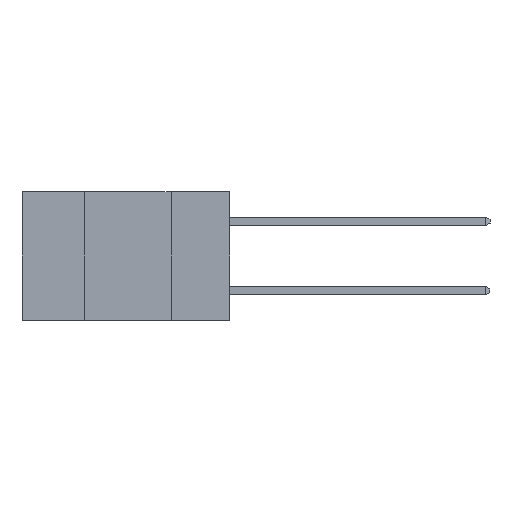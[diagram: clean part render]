
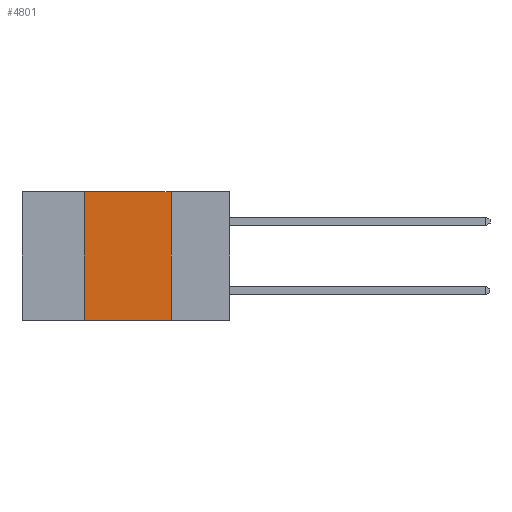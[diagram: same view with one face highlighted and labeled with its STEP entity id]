
A CAD part, left-side view. The second image highlights one B-rep face of the part: STEP entity #4801.
In plain terms, the highlighted planar face has unit normal (-1, 0, 0).
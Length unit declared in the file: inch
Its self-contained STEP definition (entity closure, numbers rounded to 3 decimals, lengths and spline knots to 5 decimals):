
#1340 = DIRECTION ( 'NONE',  ( 0., 0., -1. ) ) ;
#1509 = FACE_OUTER_BOUND ( 'NONE', #3841, .T. ) ;
#3841 = EDGE_LOOP ( 'NONE', ( #6502, #13847, #8459, #9207 ) ) ;
#3978 = VECTOR ( 'NONE', #1340, 39.37008 ) ;
#4552 = LINE ( 'NONE', #22559, #3978 ) ;
#4801 = ADVANCED_FACE ( 'NONE', ( #1509 ), #14738, .F. ) ;
#5911 = DIRECTION ( 'NONE',  ( 0., 0., 1. ) ) ;
#6206 = VERTEX_POINT ( 'NONE', #13933 ) ;
#6502 = ORIENTED_EDGE ( 'NONE', *, *, #14186, .F. ) ;
#7762 = CARTESIAN_POINT ( 'NONE',  ( 0., 0.42, -0.37 ) ) ;
#8459 = ORIENTED_EDGE ( 'NONE', *, *, #12145, .F. ) ;
#8888 = AXIS2_PLACEMENT_3D ( 'NONE', #14660, #15686, #22134 ) ;
#8908 = LINE ( 'NONE', #13937, #13091 ) ;
#9137 = CARTESIAN_POINT ( 'NONE',  ( 0., 0.17, 0. ) ) ;
#9207 = ORIENTED_EDGE ( 'NONE', *, *, #18111, .T. ) ;
#10358 = CARTESIAN_POINT ( 'NONE',  ( 0., 0.42, 0. ) ) ;
#10503 = VERTEX_POINT ( 'NONE', #10358 ) ;
#10595 = EDGE_CURVE ( 'NONE', #10503, #22707, #19248, .T. ) ;
#12145 = EDGE_CURVE ( 'NONE', #13924, #10503, #13664, .T. ) ;
#12261 = DIRECTION ( 'NONE',  ( 0., -1., 0. ) ) ;
#13091 = VECTOR ( 'NONE', #12261, 39.37008 ) ;
#13664 = LINE ( 'NONE', #20096, #17794 ) ;
#13847 = ORIENTED_EDGE ( 'NONE', *, *, #10595, .F. ) ;
#13924 = VERTEX_POINT ( 'NONE', #7762 ) ;
#13933 = CARTESIAN_POINT ( 'NONE',  ( 0., 0.17, -0.37 ) ) ;
#13937 = CARTESIAN_POINT ( 'NONE',  ( 0., 0.6, -0.37 ) ) ;
#14027 = VECTOR ( 'NONE', #22747, 39.37008 ) ;
#14186 = EDGE_CURVE ( 'NONE', #22707, #6206, #4552, .T. ) ;
#14660 = CARTESIAN_POINT ( 'NONE',  ( 0., 0.6, 0. ) ) ;
#14738 = PLANE ( 'NONE',  #8888 ) ;
#15686 = DIRECTION ( 'NONE',  ( 1., 0., 0. ) ) ;
#15828 = CARTESIAN_POINT ( 'NONE',  ( 0., 0.6, 0. ) ) ;
#17794 = VECTOR ( 'NONE', #5911, 39.37008 ) ;
#18111 = EDGE_CURVE ( 'NONE', #13924, #6206, #8908, .T. ) ;
#19248 = LINE ( 'NONE', #15828, #14027 ) ;
#20096 = CARTESIAN_POINT ( 'NONE',  ( 0., 0.42, 0. ) ) ;
#22134 = DIRECTION ( 'NONE',  ( 0., 0., -1. ) ) ;
#22559 = CARTESIAN_POINT ( 'NONE',  ( 0., 0.17, 0. ) ) ;
#22707 = VERTEX_POINT ( 'NONE', #9137 ) ;
#22747 = DIRECTION ( 'NONE',  ( 0., -1., 0. ) ) ;
